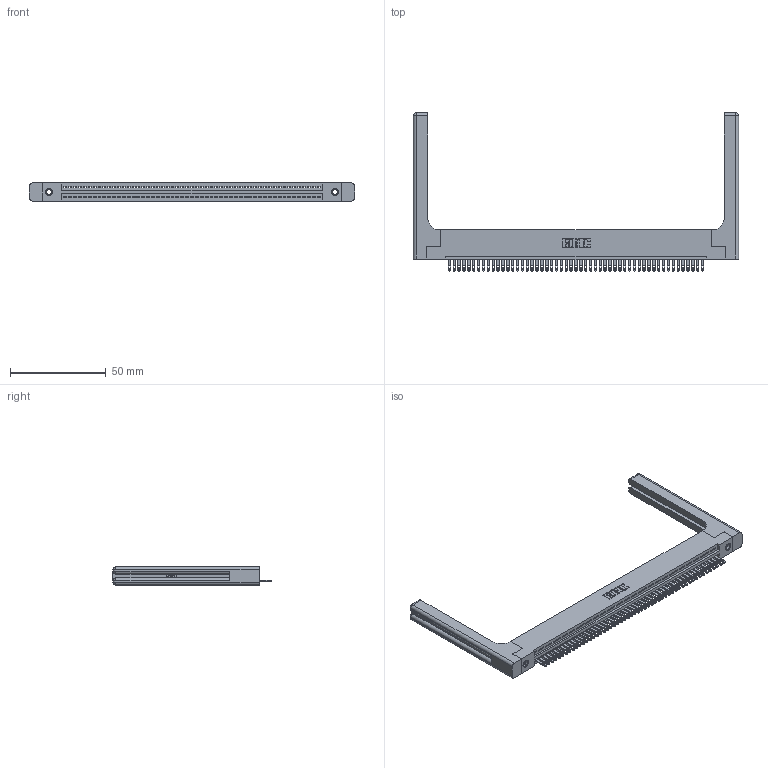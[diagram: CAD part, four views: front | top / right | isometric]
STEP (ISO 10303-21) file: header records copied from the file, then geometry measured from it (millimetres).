
FILE_DESCRIPTION (( 'STEP AP203' ), '1' );
FILE_NAME ('345-053-500-158.STEP', '2019-10-09T19:48:20', ( '' ), ( '' ), 'SwSTEP 2.0', 'SolidWorks 2016', '' );
FILE_SCHEMA (( 'CONFIG_CONTROL_DESIGN' ));
Length unit declared in the file: inch
Products named in the file (5): 345-053-500-158; 345 Part_Flush Mounting Lugs - 0.156 Dia-TH; 345-220-058_345-220-058; 345-250-001_345-250-001-102; 345-292-001_345-293-100
Assembly tree (58 placements, depth 2):
  345-053-500-158
    345 Part_Flush Mounting Lugs - 0.156 Dia-TH
    345-292-001_345-293-100  x53
    345-250-001_345-250-001-102  x2
    345-220-058_345-220-058  x2
Bounding box: 169.65 x 82.47 x 9.4 mm (x, y, z)
Volume: 24741.1 mm3; surface area: 27150.4 mm2
Topology: 58 solids, 58 shells, 3244 faces, 9911 edges, 6586 vertices
Faces by surface type: plane 2030, cylinder 1154, bspline 36, cone 12, sphere 8, torus 4
Entity records: 43520 total; most frequent: CARTESIAN_POINT 8508, ORIENTED_EDGE 7292, DIRECTION 6364, EDGE_CURVE 3646, LINE 3206, VECTOR 3206, VERTEX_POINT 2422, AXIS2_PLACEMENT_3D 1579
